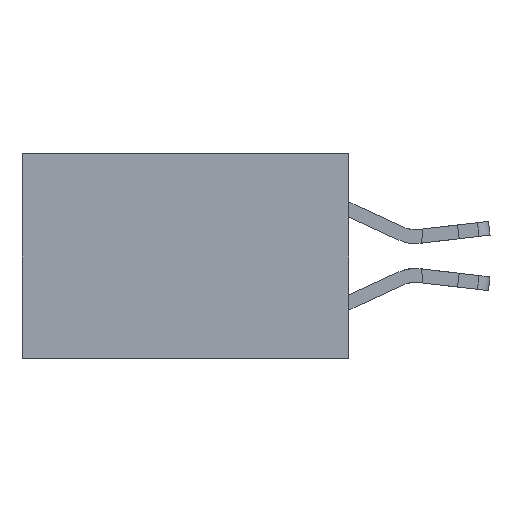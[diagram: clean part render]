
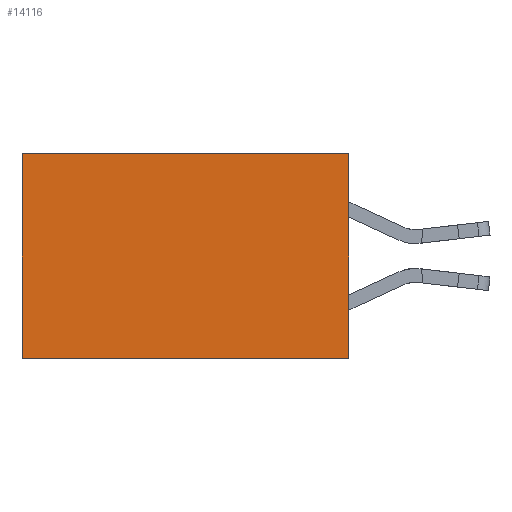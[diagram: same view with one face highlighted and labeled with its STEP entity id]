
A CAD part, left-side view. The second image highlights one B-rep face of the part: STEP entity #14116.
In plain terms, the highlighted planar face has unit normal (-1, 0, 0).
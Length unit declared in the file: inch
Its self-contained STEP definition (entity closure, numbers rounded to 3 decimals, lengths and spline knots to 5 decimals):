
#77 = VECTOR ( 'NONE', #10346, 39.37008 ) ;
#567 = VECTOR ( 'NONE', #20149, 39.37008 ) ;
#1042 = VECTOR ( 'NONE', #17462, 39.37008 ) ;
#2053 = DIRECTION ( 'NONE',  ( 1., 0., 0. ) ) ;
#2056 = LINE ( 'NONE', #10583, #77 ) ;
#2556 = DIRECTION ( 'NONE',  ( 0., 1., 0. ) ) ;
#2726 = FACE_OUTER_BOUND ( 'NONE', #23945, .T. ) ;
#3110 = VECTOR ( 'NONE', #2556, 39.37008 ) ;
#5304 = ORIENTED_EDGE ( 'NONE', *, *, #21906, .F. ) ;
#5385 = CARTESIAN_POINT ( 'NONE',  ( 0.277, 0.59, -0.37 ) ) ;
#8307 = EDGE_CURVE ( 'NONE', #8377, #25632, #11617, .T. ) ;
#8377 = VERTEX_POINT ( 'NONE', #16566 ) ;
#8844 = EDGE_CURVE ( 'NONE', #10287, #8377, #2056, .T. ) ;
#9393 = LINE ( 'NONE', #23165, #3110 ) ;
#9475 = ORIENTED_EDGE ( 'NONE', *, *, #20252, .F. ) ;
#10287 = VERTEX_POINT ( 'NONE', #25136 ) ;
#10346 = DIRECTION ( 'NONE',  ( 0., 1., 0. ) ) ;
#10583 = CARTESIAN_POINT ( 'NONE',  ( 0.277, 0., 0. ) ) ;
#10756 = VERTEX_POINT ( 'NONE', #16728 ) ;
#11617 = LINE ( 'NONE', #17808, #1042 ) ;
#11767 = LINE ( 'NONE', #18159, #567 ) ;
#14116 = ADVANCED_FACE ( 'NONE', ( #2726 ), #19594, .F. ) ;
#14676 = CARTESIAN_POINT ( 'NONE',  ( 0.277, 0., -0.37 ) ) ;
#16566 = CARTESIAN_POINT ( 'NONE',  ( 0.277, 0.59, 0. ) ) ;
#16728 = CARTESIAN_POINT ( 'NONE',  ( 0.277, 0., -0.37 ) ) ;
#16750 = DIRECTION ( 'NONE',  ( 0., 0., -1. ) ) ;
#17462 = DIRECTION ( 'NONE',  ( 0., 0., -1. ) ) ;
#17620 = ORIENTED_EDGE ( 'NONE', *, *, #8844, .T. ) ;
#17808 = CARTESIAN_POINT ( 'NONE',  ( 0.277, 0.59, -0.37 ) ) ;
#18159 = CARTESIAN_POINT ( 'NONE',  ( 0.277, 0., -0.37 ) ) ;
#19594 = PLANE ( 'NONE',  #25825 ) ;
#20149 = DIRECTION ( 'NONE',  ( 0., 0., -1. ) ) ;
#20252 = EDGE_CURVE ( 'NONE', #10287, #10756, #11767, .T. ) ;
#21906 = EDGE_CURVE ( 'NONE', #10756, #25632, #9393, .T. ) ;
#23165 = CARTESIAN_POINT ( 'NONE',  ( 0.277, 0., -0.37 ) ) ;
#23682 = ORIENTED_EDGE ( 'NONE', *, *, #8307, .T. ) ;
#23945 = EDGE_LOOP ( 'NONE', ( #23682, #5304, #9475, #17620 ) ) ;
#25136 = CARTESIAN_POINT ( 'NONE',  ( 0.277, 0., 0. ) ) ;
#25632 = VERTEX_POINT ( 'NONE', #5385 ) ;
#25825 = AXIS2_PLACEMENT_3D ( 'NONE', #14676, #2053, #16750 ) ;
